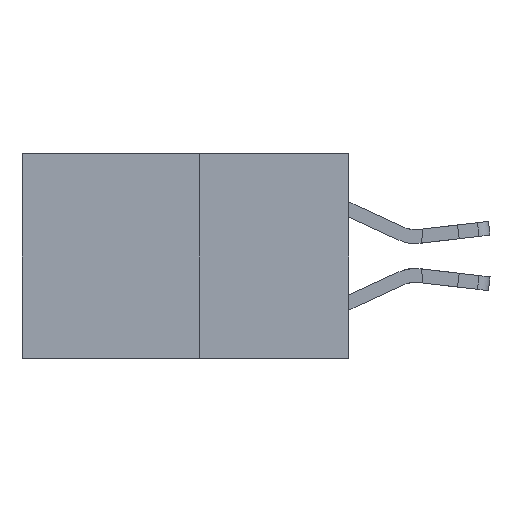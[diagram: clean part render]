
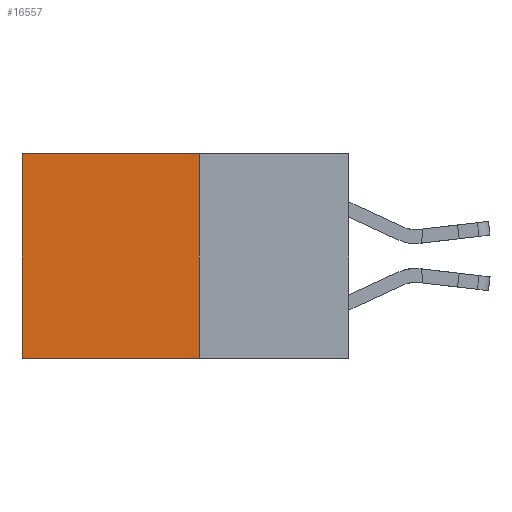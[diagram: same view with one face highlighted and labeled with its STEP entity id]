
A CAD part, left-side view. The second image highlights one B-rep face of the part: STEP entity #16557.
In plain terms, the highlighted planar face has unit normal (-1, 0, 0).
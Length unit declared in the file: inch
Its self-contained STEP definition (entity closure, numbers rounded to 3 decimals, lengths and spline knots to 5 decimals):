
#437 = CARTESIAN_POINT ( 'NONE',  ( 0.277, 0.27, -0.37 ) ) ;
#905 = EDGE_CURVE ( 'NONE', #21469, #18344, #4396, .T. ) ;
#1425 = FACE_OUTER_BOUND ( 'NONE', #7664, .T. ) ;
#2072 = LINE ( 'NONE', #21565, #21037 ) ;
#2535 = DIRECTION ( 'NONE',  ( 1., 0., 0. ) ) ;
#4396 = LINE ( 'NONE', #11734, #13607 ) ;
#4975 = EDGE_CURVE ( 'NONE', #18344, #17093, #14313, .T. ) ;
#4979 = LINE ( 'NONE', #17350, #19049 ) ;
#6630 = ORIENTED_EDGE ( 'NONE', *, *, #21346, .F. ) ;
#7664 = EDGE_LOOP ( 'NONE', ( #12316, #6630, #11300, #23451 ) ) ;
#7743 = VERTEX_POINT ( 'NONE', #437 ) ;
#9471 = CARTESIAN_POINT ( 'NONE',  ( 0.277, 0.59, -0.37 ) ) ;
#9654 = DIRECTION ( 'NONE',  ( 0., 0., -1. ) ) ;
#11300 = ORIENTED_EDGE ( 'NONE', *, *, #12560, .F. ) ;
#11734 = CARTESIAN_POINT ( 'NONE',  ( 0.277, 0.27, 0. ) ) ;
#12316 = ORIENTED_EDGE ( 'NONE', *, *, #4975, .T. ) ;
#12560 = EDGE_CURVE ( 'NONE', #21469, #7743, #4979, .T. ) ;
#13188 = CARTESIAN_POINT ( 'NONE',  ( 0.277, 0.59, -0.37 ) ) ;
#13607 = VECTOR ( 'NONE', #18119, 39.37008 ) ;
#13661 = DIRECTION ( 'NONE',  ( 0., 0., -1. ) ) ;
#14313 = LINE ( 'NONE', #9471, #19179 ) ;
#14826 = CARTESIAN_POINT ( 'NONE',  ( 0.277, 0.59, 0. ) ) ;
#15279 = CARTESIAN_POINT ( 'NONE',  ( 0.277, 0.27, -0.37 ) ) ;
#15355 = DIRECTION ( 'NONE',  ( 0., 0., -1. ) ) ;
#16557 = ADVANCED_FACE ( 'NONE', ( #1425 ), #22712, .F. ) ;
#17093 = VERTEX_POINT ( 'NONE', #13188 ) ;
#17350 = CARTESIAN_POINT ( 'NONE',  ( 0.277, 0.27, -0.37 ) ) ;
#17910 = DIRECTION ( 'NONE',  ( 0., 1., 0. ) ) ;
#18119 = DIRECTION ( 'NONE',  ( 0., 1., 0. ) ) ;
#18344 = VERTEX_POINT ( 'NONE', #14826 ) ;
#19049 = VECTOR ( 'NONE', #13661, 39.37008 ) ;
#19179 = VECTOR ( 'NONE', #9654, 39.37008 ) ;
#19501 = AXIS2_PLACEMENT_3D ( 'NONE', #15279, #2535, #15355 ) ;
#21037 = VECTOR ( 'NONE', #17910, 39.37008 ) ;
#21346 = EDGE_CURVE ( 'NONE', #7743, #17093, #2072, .T. ) ;
#21469 = VERTEX_POINT ( 'NONE', #21945 ) ;
#21565 = CARTESIAN_POINT ( 'NONE',  ( 0.277, 0.27, -0.37 ) ) ;
#21945 = CARTESIAN_POINT ( 'NONE',  ( 0.277, 0.27, 0. ) ) ;
#22712 = PLANE ( 'NONE',  #19501 ) ;
#23451 = ORIENTED_EDGE ( 'NONE', *, *, #905, .T. ) ;
